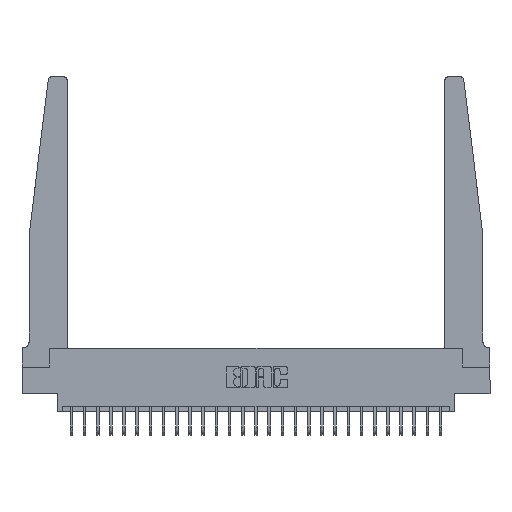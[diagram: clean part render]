
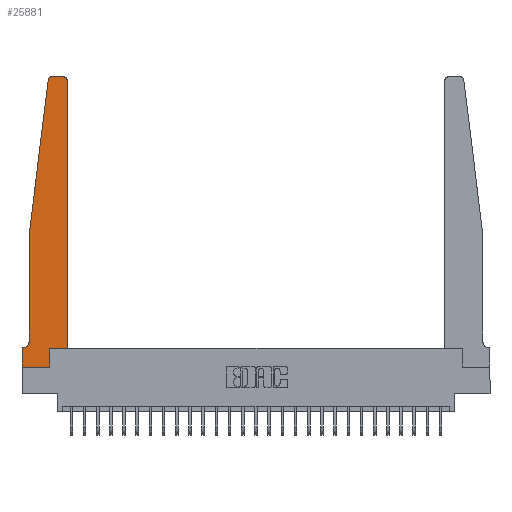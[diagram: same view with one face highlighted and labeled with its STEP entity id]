
A CAD part, top view. The second image highlights one B-rep face of the part: STEP entity #25881.
In plain terms, the highlighted planar face has unit normal (0, 0, 1).
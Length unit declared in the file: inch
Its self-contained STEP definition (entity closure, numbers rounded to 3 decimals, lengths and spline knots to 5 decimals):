
#213 = DIRECTION ( 'NONE',  ( 1., 0., 0. ) ) ;
#330 = EDGE_CURVE ( 'NONE', #13837, #19894, #26229, .T. ) ;
#538 = CARTESIAN_POINT ( 'NONE',  ( 0.065, 0.1875, 0.37 ) ) ;
#652 = CARTESIAN_POINT ( 'NONE',  ( 0.395, 2.75, 0.37 ) ) ;
#1071 = PLANE ( 'NONE',  #12837 ) ;
#1379 = VECTOR ( 'NONE', #14681, 39.37008 ) ;
#1593 = EDGE_CURVE ( 'NONE', #2897, #26255, #24933, .T. ) ;
#1673 = EDGE_CURVE ( 'NONE', #16791, #18307, #20564, .T. ) ;
#1861 = CARTESIAN_POINT ( 'NONE',  ( 0.065, 1.25, 0.37 ) ) ;
#2340 = EDGE_CURVE ( 'NONE', #26255, #14648, #24039, .T. ) ;
#2600 = ORIENTED_EDGE ( 'NONE', *, *, #2340, .T. ) ;
#2897 = VERTEX_POINT ( 'NONE', #9287 ) ;
#3017 = ORIENTED_EDGE ( 'NONE', *, *, #1673, .T. ) ;
#3067 = DIRECTION ( 'NONE',  ( 0., 0., 1. ) ) ;
#3186 = CARTESIAN_POINT ( 'NONE',  ( 0.425, 0.18, 0.37 ) ) ;
#3312 = FACE_OUTER_BOUND ( 'NONE', #27231, .T. ) ;
#4892 = DIRECTION ( 'NONE',  ( -1., 0., 0. ) ) ;
#5220 = ORIENTED_EDGE ( 'NONE', *, *, #19453, .T. ) ;
#5423 = DIRECTION ( 'NONE',  ( 1., 0., 0. ) ) ;
#5435 = EDGE_CURVE ( 'NONE', #18307, #2897, #12551, .T. ) ;
#5790 = DIRECTION ( 'NONE',  ( 1., 0., 0. ) ) ;
#6258 = VERTEX_POINT ( 'NONE', #22073 ) ;
#6739 = EDGE_CURVE ( 'NONE', #6258, #9536, #22442, .T. ) ;
#6934 = DIRECTION ( 'NONE',  ( 0., 1., 0. ) ) ;
#7615 = ORIENTED_EDGE ( 'NONE', *, *, #5435, .T. ) ;
#7680 = CARTESIAN_POINT ( 'NONE',  ( 0.25, 2.75, 0.37 ) ) ;
#7732 = CIRCLE ( 'NONE', #14001, 0.03 ) ;
#7956 = EDGE_CURVE ( 'NONE', #27118, #25105, #11892, .T. ) ;
#7960 = DIRECTION ( 'NONE',  ( 1., 0., 0. ) ) ;
#8500 = DIRECTION ( 'NONE',  ( 0., 0., 1. ) ) ;
#8592 = VECTOR ( 'NONE', #22176, 39.37008 ) ;
#8645 = CARTESIAN_POINT ( 'NONE',  ( 0.395, 2.72, 0.37 ) ) ;
#8767 = VECTOR ( 'NONE', #7960, 39.37008 ) ;
#9190 = CARTESIAN_POINT ( 'NONE',  ( 0.015, 0.1875, 0.37 ) ) ;
#9287 = CARTESIAN_POINT ( 'NONE',  ( 0.065, 0.2375, 0.37 ) ) ;
#9444 = DIRECTION ( 'NONE',  ( 0., 0., -1. ) ) ;
#9536 = VERTEX_POINT ( 'NONE', #26916 ) ;
#9781 = LINE ( 'NONE', #20618, #8767 ) ;
#11078 = CARTESIAN_POINT ( 'NONE',  ( 0.27653, 2.75, 0.37 ) ) ;
#11174 = ORIENTED_EDGE ( 'NONE', *, *, #6739, .T. ) ;
#11315 = CARTESIAN_POINT ( 'NONE',  ( 0., 0.1875, 0.37 ) ) ;
#11399 = VECTOR ( 'NONE', #16640, 39.37008 ) ;
#11741 = DIRECTION ( 'NONE',  ( 0., 1., 0. ) ) ;
#11758 = DIRECTION ( 'NONE',  ( 1., 0., 0. ) ) ;
#11892 = LINE ( 'NONE', #7680, #8592 ) ;
#12551 = LINE ( 'NONE', #19034, #11399 ) ;
#12837 = AXIS2_PLACEMENT_3D ( 'NONE', #11315, #24419, #5423 ) ;
#13120 = CARTESIAN_POINT ( 'NONE',  ( 0.065, 1.25, 0.37 ) ) ;
#13837 = VERTEX_POINT ( 'NONE', #17892 ) ;
#13933 = CARTESIAN_POINT ( 'NONE',  ( 0.24675, 2.72367, 0.37 ) ) ;
#14001 = AXIS2_PLACEMENT_3D ( 'NONE', #8645, #8500, #213 ) ;
#14529 = VECTOR ( 'NONE', #5790, 39.37008 ) ;
#14648 = VERTEX_POINT ( 'NONE', #17961 ) ;
#14681 = DIRECTION ( 'NONE',  ( 0., -1., 0. ) ) ;
#15141 = VERTEX_POINT ( 'NONE', #24143 ) ;
#15518 = CARTESIAN_POINT ( 'NONE',  ( 0.2605, 0.18, 0.37 ) ) ;
#16406 = AXIS2_PLACEMENT_3D ( 'NONE', #18246, #3067, #11758 ) ;
#16484 = DIRECTION ( 'NONE',  ( -0.122, -0.992, 0. ) ) ;
#16640 = DIRECTION ( 'NONE',  ( 0., -1., 0. ) ) ;
#16791 = VERTEX_POINT ( 'NONE', #13933 ) ;
#16855 = VECTOR ( 'NONE', #4892, 39.37008 ) ;
#16949 = VECTOR ( 'NONE', #6934, 39.37008 ) ;
#17746 = CIRCLE ( 'NONE', #16406, 0.03 ) ;
#17892 = CARTESIAN_POINT ( 'NONE',  ( 0.2605, 0., 0.37 ) ) ;
#17961 = CARTESIAN_POINT ( 'NONE',  ( 0., 0.1875, 0.37 ) ) ;
#18029 = DIRECTION ( 'NONE',  ( -1., 0., 0. ) ) ;
#18185 = VECTOR ( 'NONE', #16484, 39.37008 ) ;
#18246 = CARTESIAN_POINT ( 'NONE',  ( 0.27653, 2.72, 0.37 ) ) ;
#18272 = ORIENTED_EDGE ( 'NONE', *, *, #23497, .T. ) ;
#18307 = VERTEX_POINT ( 'NONE', #13120 ) ;
#18425 = LINE ( 'NONE', #22931, #14529 ) ;
#18737 = CARTESIAN_POINT ( 'NONE',  ( 0.2605, 0.18, 0.37 ) ) ;
#18751 = ORIENTED_EDGE ( 'NONE', *, *, #24399, .T. ) ;
#18905 = LINE ( 'NONE', #27793, #1379 ) ;
#19034 = CARTESIAN_POINT ( 'NONE',  ( 0.065, 1.25, 0.37 ) ) ;
#19036 = ORIENTED_EDGE ( 'NONE', *, *, #1593, .T. ) ;
#19095 = ORIENTED_EDGE ( 'NONE', *, *, #330, .T. ) ;
#19453 = EDGE_CURVE ( 'NONE', #14648, #15141, #18905, .T. ) ;
#19894 = VERTEX_POINT ( 'NONE', #18737 ) ;
#20289 = CARTESIAN_POINT ( 'NONE',  ( 0.015, 0.2375, 0.37 ) ) ;
#20368 = ORIENTED_EDGE ( 'NONE', *, *, #25334, .T. ) ;
#20564 = LINE ( 'NONE', #1861, #18185 ) ;
#20618 = CARTESIAN_POINT ( 'NONE',  ( 0.425, 0.18, 0.37 ) ) ;
#21363 = EDGE_CURVE ( 'NONE', #9536, #27118, #7732, .T. ) ;
#21455 = VECTOR ( 'NONE', #11741, 39.37008 ) ;
#22073 = CARTESIAN_POINT ( 'NONE',  ( 0.425, 0.18, 0.37 ) ) ;
#22176 = DIRECTION ( 'NONE',  ( -1., 0., 0. ) ) ;
#22442 = LINE ( 'NONE', #3186, #21455 ) ;
#22931 = CARTESIAN_POINT ( 'NONE',  ( 0., 0., 0.37 ) ) ;
#23497 = EDGE_CURVE ( 'NONE', #15141, #13837, #18425, .T. ) ;
#24039 = LINE ( 'NONE', #538, #16855 ) ;
#24143 = CARTESIAN_POINT ( 'NONE',  ( 0., 0., 0.37 ) ) ;
#24399 = EDGE_CURVE ( 'NONE', #19894, #6258, #9781, .T. ) ;
#24413 = ORIENTED_EDGE ( 'NONE', *, *, #7956, .T. ) ;
#24419 = DIRECTION ( 'NONE',  ( 0., 0., 1. ) ) ;
#24933 = CIRCLE ( 'NONE', #27194, 0.05 ) ;
#25105 = VERTEX_POINT ( 'NONE', #11078 ) ;
#25334 = EDGE_CURVE ( 'NONE', #25105, #16791, #17746, .T. ) ;
#25744 = ORIENTED_EDGE ( 'NONE', *, *, #21363, .T. ) ;
#25881 = ADVANCED_FACE ( 'NONE', ( #3312 ), #1071, .T. ) ;
#26229 = LINE ( 'NONE', #15518, #16949 ) ;
#26255 = VERTEX_POINT ( 'NONE', #9190 ) ;
#26916 = CARTESIAN_POINT ( 'NONE',  ( 0.425, 2.72, 0.37 ) ) ;
#27118 = VERTEX_POINT ( 'NONE', #652 ) ;
#27194 = AXIS2_PLACEMENT_3D ( 'NONE', #20289, #9444, #18029 ) ;
#27231 = EDGE_LOOP ( 'NONE', ( #24413, #20368, #3017, #7615, #19036, #2600, #5220, #18272, #19095, #18751, #11174, #25744 ) ) ;
#27793 = CARTESIAN_POINT ( 'NONE',  ( 0., 0., 0.37 ) ) ;
